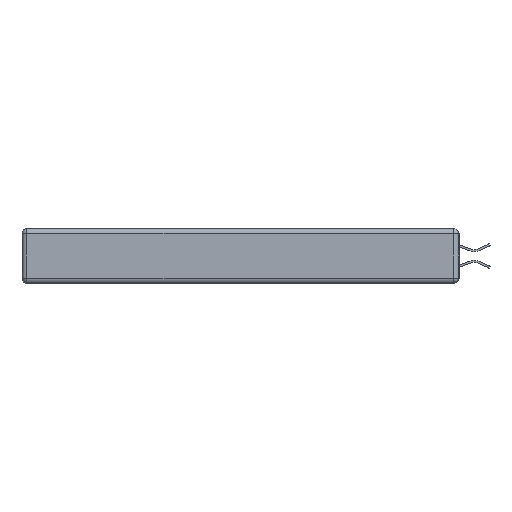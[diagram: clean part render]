
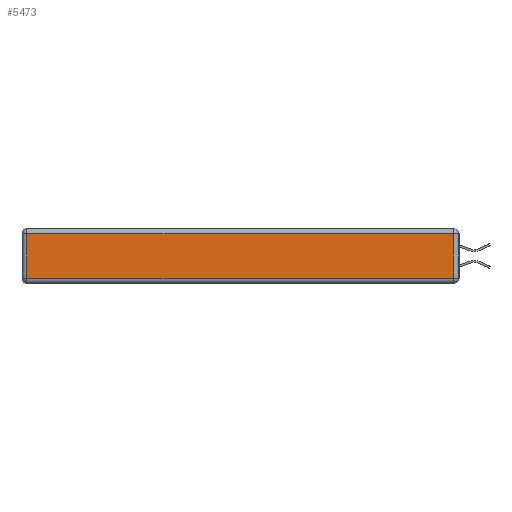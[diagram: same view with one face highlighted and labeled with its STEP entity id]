
A CAD part, left-side view. The second image highlights one B-rep face of the part: STEP entity #5473.
In plain terms, the highlighted planar face has unit normal (-1, 0, 0).
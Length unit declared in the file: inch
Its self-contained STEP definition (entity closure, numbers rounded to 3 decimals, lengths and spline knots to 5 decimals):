
#260 = AXIS2_PLACEMENT_3D ( 'NONE', #11903, #11139, #5425 ) ;
#576 = ORIENTED_EDGE ( 'NONE', *, *, #3130, .T. ) ;
#829 = VECTOR ( 'NONE', #10802, 39.37008 ) ;
#2349 = ORIENTED_EDGE ( 'NONE', *, *, #6507, .T. ) ;
#3130 = EDGE_CURVE ( 'NONE', #14396, #6767, #7635, .T. ) ;
#3883 = LINE ( 'NONE', #11889, #829 ) ;
#3903 = PLANE ( 'NONE',  #260 ) ;
#4354 = VECTOR ( 'NONE', #10155, 39.37008 ) ;
#4803 = CARTESIAN_POINT ( 'NONE',  ( 0., 2.72, -0.313 ) ) ;
#4939 = LINE ( 'NONE', #13481, #7996 ) ;
#5425 = DIRECTION ( 'NONE',  ( 0., 0., 1. ) ) ;
#5473 = ADVANCED_FACE ( 'NONE', ( #12330 ), #3903, .T. ) ;
#6131 = EDGE_CURVE ( 'NONE', #13284, #6537, #4939, .T. ) ;
#6283 = LINE ( 'NONE', #6725, #4354 ) ;
#6488 = CARTESIAN_POINT ( 'NONE',  ( 0., 2.75, -0.03 ) ) ;
#6507 = EDGE_CURVE ( 'NONE', #6537, #14396, #3883, .T. ) ;
#6537 = VERTEX_POINT ( 'NONE', #10906 ) ;
#6725 = CARTESIAN_POINT ( 'NONE',  ( 0., 2.72, -0.343 ) ) ;
#6767 = VERTEX_POINT ( 'NONE', #10813 ) ;
#6908 = DIRECTION ( 'NONE',  ( 0., -1., 0. ) ) ;
#7635 = LINE ( 'NONE', #6488, #14458 ) ;
#7979 = ORIENTED_EDGE ( 'NONE', *, *, #9830, .T. ) ;
#7996 = VECTOR ( 'NONE', #6908, 39.37008 ) ;
#9830 = EDGE_CURVE ( 'NONE', #6767, #13284, #6283, .T. ) ;
#10155 = DIRECTION ( 'NONE',  ( 0., 0., -1. ) ) ;
#10802 = DIRECTION ( 'NONE',  ( 0., 0., 1. ) ) ;
#10813 = CARTESIAN_POINT ( 'NONE',  ( 0., 2.72, -0.03 ) ) ;
#10906 = CARTESIAN_POINT ( 'NONE',  ( 0., 0.03, -0.313 ) ) ;
#11139 = DIRECTION ( 'NONE',  ( -1., 0., 0. ) ) ;
#11692 = ORIENTED_EDGE ( 'NONE', *, *, #6131, .T. ) ;
#11889 = CARTESIAN_POINT ( 'NONE',  ( 0., 0.03, -0.343 ) ) ;
#11903 = CARTESIAN_POINT ( 'NONE',  ( 0., 0., -0.343 ) ) ;
#12330 = FACE_OUTER_BOUND ( 'NONE', #12575, .T. ) ;
#12416 = DIRECTION ( 'NONE',  ( 0., 1., 0. ) ) ;
#12575 = EDGE_LOOP ( 'NONE', ( #11692, #2349, #576, #7979 ) ) ;
#13284 = VERTEX_POINT ( 'NONE', #4803 ) ;
#13481 = CARTESIAN_POINT ( 'NONE',  ( 0., 0., -0.313 ) ) ;
#13701 = CARTESIAN_POINT ( 'NONE',  ( 0., 0.03, -0.03 ) ) ;
#14396 = VERTEX_POINT ( 'NONE', #13701 ) ;
#14458 = VECTOR ( 'NONE', #12416, 39.37008 ) ;
